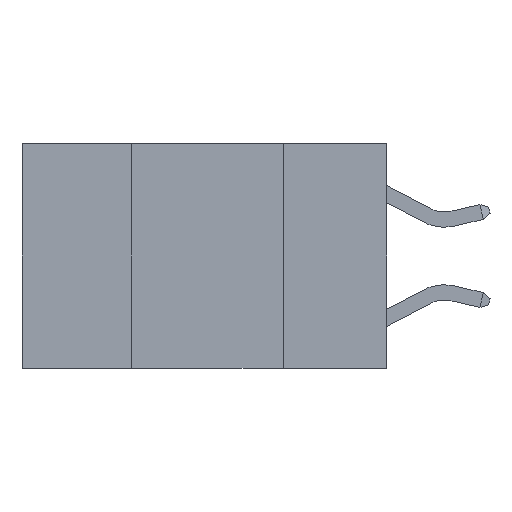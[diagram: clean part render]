
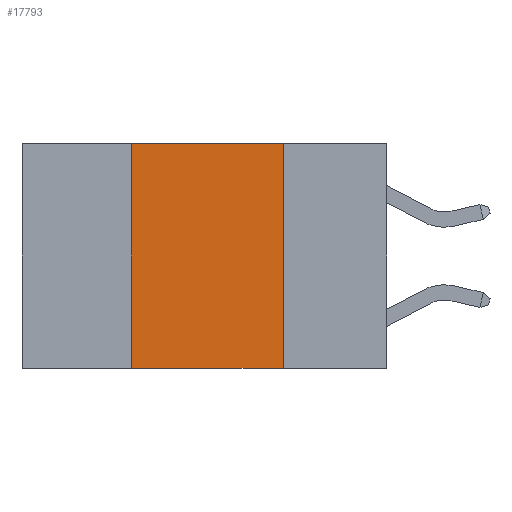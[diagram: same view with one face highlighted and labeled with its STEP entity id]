
A CAD part, left-side view. The second image highlights one B-rep face of the part: STEP entity #17793.
In plain terms, the highlighted planar face has unit normal (-1, 0, 0).
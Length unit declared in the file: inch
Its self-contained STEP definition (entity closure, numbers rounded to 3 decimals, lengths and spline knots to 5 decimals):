
#4 = CARTESIAN_POINT ( 'NONE',  ( 0., 0.17, -0.37 ) ) ;
#255 = ORIENTED_EDGE ( 'NONE', *, *, #26424, .T. ) ;
#790 = CARTESIAN_POINT ( 'NONE',  ( 0., 0.17, 0. ) ) ;
#1309 = ORIENTED_EDGE ( 'NONE', *, *, #1605, .F. ) ;
#1605 = EDGE_CURVE ( 'NONE', #26312, #5690, #18855, .T. ) ;
#3132 = DIRECTION ( 'NONE',  ( 1., 0., 0. ) ) ;
#3379 = CARTESIAN_POINT ( 'NONE',  ( 0., 0.6, -0.37 ) ) ;
#3804 = LINE ( 'NONE', #24706, #28181 ) ;
#5690 = VERTEX_POINT ( 'NONE', #790 ) ;
#6072 = VERTEX_POINT ( 'NONE', #4 ) ;
#7350 = FACE_OUTER_BOUND ( 'NONE', #20639, .T. ) ;
#7408 = VECTOR ( 'NONE', #19151, 39.37008 ) ;
#7905 = CARTESIAN_POINT ( 'NONE',  ( 0., 0.42, 0. ) ) ;
#8014 = LINE ( 'NONE', #15109, #9915 ) ;
#8554 = AXIS2_PLACEMENT_3D ( 'NONE', #16543, #3132, #9778 ) ;
#9778 = DIRECTION ( 'NONE',  ( 0., 0., -1. ) ) ;
#9915 = VECTOR ( 'NONE', #13146, 39.37008 ) ;
#10305 = LINE ( 'NONE', #3379, #17362 ) ;
#12036 = PLANE ( 'NONE',  #8554 ) ;
#12540 = DIRECTION ( 'NONE',  ( 0., 0., 1. ) ) ;
#13146 = DIRECTION ( 'NONE',  ( 0., 0., -1. ) ) ;
#14405 = ORIENTED_EDGE ( 'NONE', *, *, #15701, .F. ) ;
#15109 = CARTESIAN_POINT ( 'NONE',  ( 0., 0.17, 0. ) ) ;
#15636 = EDGE_CURVE ( 'NONE', #17336, #26312, #3804, .T. ) ;
#15701 = EDGE_CURVE ( 'NONE', #5690, #6072, #8014, .T. ) ;
#16543 = CARTESIAN_POINT ( 'NONE',  ( 0., 0.6, 0. ) ) ;
#17336 = VERTEX_POINT ( 'NONE', #26059 ) ;
#17362 = VECTOR ( 'NONE', #26722, 39.37008 ) ;
#17793 = ADVANCED_FACE ( 'NONE', ( #7350 ), #12036, .F. ) ;
#18855 = LINE ( 'NONE', #28657, #7408 ) ;
#19151 = DIRECTION ( 'NONE',  ( 0., -1., 0. ) ) ;
#19748 = ORIENTED_EDGE ( 'NONE', *, *, #15636, .F. ) ;
#20639 = EDGE_LOOP ( 'NONE', ( #14405, #1309, #19748, #255 ) ) ;
#24706 = CARTESIAN_POINT ( 'NONE',  ( 0., 0.42, 0. ) ) ;
#26059 = CARTESIAN_POINT ( 'NONE',  ( 0., 0.42, -0.37 ) ) ;
#26312 = VERTEX_POINT ( 'NONE', #7905 ) ;
#26424 = EDGE_CURVE ( 'NONE', #17336, #6072, #10305, .T. ) ;
#26722 = DIRECTION ( 'NONE',  ( 0., -1., 0. ) ) ;
#28181 = VECTOR ( 'NONE', #12540, 39.37008 ) ;
#28657 = CARTESIAN_POINT ( 'NONE',  ( 0., 0.6, 0. ) ) ;
